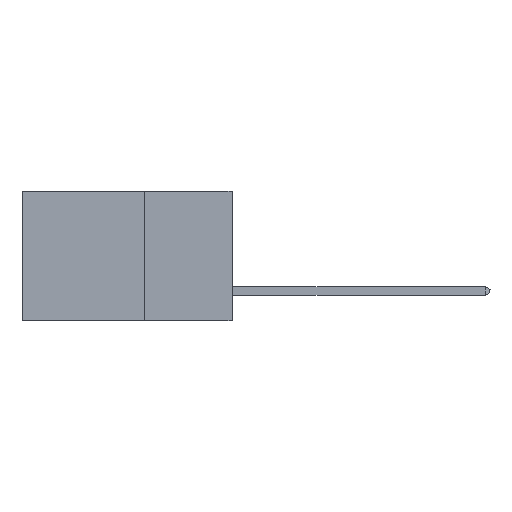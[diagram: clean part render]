
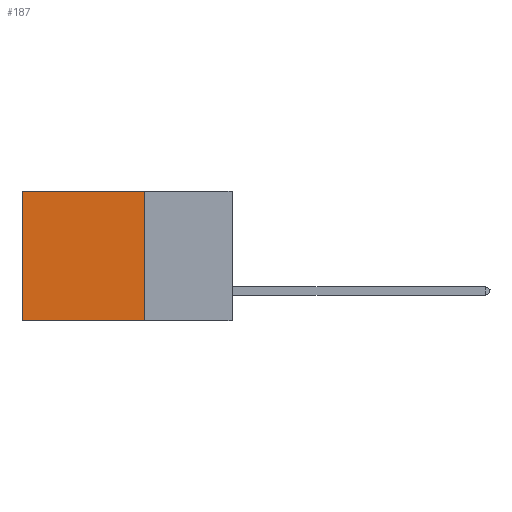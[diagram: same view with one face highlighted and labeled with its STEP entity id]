
A CAD part, left-side view. The second image highlights one B-rep face of the part: STEP entity #187.
In plain terms, the highlighted planar face has unit normal (-1, 0, 0).
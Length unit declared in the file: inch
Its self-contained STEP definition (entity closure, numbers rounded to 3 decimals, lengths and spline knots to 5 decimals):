
#187 = ADVANCED_FACE ( 'NONE', ( #5172 ), #18684, .F. ) ;
#511 = ORIENTED_EDGE ( 'NONE', *, *, #18909, .F. ) ;
#770 = VECTOR ( 'NONE', #10409, 39.37008 ) ;
#1009 = VECTOR ( 'NONE', #8245, 39.37008 ) ;
#1285 = CARTESIAN_POINT ( 'NONE',  ( 0.2875, 0.6, 0. ) ) ;
#1453 = CARTESIAN_POINT ( 'NONE',  ( 0.2875, 0.25, 0. ) ) ;
#2769 = VERTEX_POINT ( 'NONE', #27573 ) ;
#3596 = ORIENTED_EDGE ( 'NONE', *, *, #14658, .T. ) ;
#3694 = DIRECTION ( 'NONE',  ( 0., 1., 0. ) ) ;
#4223 = CARTESIAN_POINT ( 'NONE',  ( 0.2875, 0.6, -0.37 ) ) ;
#4776 = LINE ( 'NONE', #6081, #27392 ) ;
#5172 = FACE_OUTER_BOUND ( 'NONE', #27755, .T. ) ;
#5697 = CARTESIAN_POINT ( 'NONE',  ( 0.2875, 0.25, 0. ) ) ;
#5830 = VECTOR ( 'NONE', #24695, 39.37008 ) ;
#6081 = CARTESIAN_POINT ( 'NONE',  ( 0.2875, 0.25, -0.37 ) ) ;
#7143 = LINE ( 'NONE', #22536, #5830 ) ;
#7458 = VERTEX_POINT ( 'NONE', #11482 ) ;
#7791 = EDGE_CURVE ( 'NONE', #2769, #12988, #4776, .T. ) ;
#7856 = CARTESIAN_POINT ( 'NONE',  ( 0.2875, 0.25, 0. ) ) ;
#8245 = DIRECTION ( 'NONE',  ( 0., 0., -1. ) ) ;
#8642 = LINE ( 'NONE', #1453, #770 ) ;
#10409 = DIRECTION ( 'NONE',  ( 0., 0., -1. ) ) ;
#11482 = CARTESIAN_POINT ( 'NONE',  ( 0.2875, 0.6, 0. ) ) ;
#12988 = VERTEX_POINT ( 'NONE', #4223 ) ;
#14193 = LINE ( 'NONE', #1285, #1009 ) ;
#14499 = AXIS2_PLACEMENT_3D ( 'NONE', #5697, #20645, #20837 ) ;
#14658 = EDGE_CURVE ( 'NONE', #15773, #7458, #7143, .T. ) ;
#15773 = VERTEX_POINT ( 'NONE', #7856 ) ;
#17794 = ORIENTED_EDGE ( 'NONE', *, *, #21390, .T. ) ;
#18684 = PLANE ( 'NONE',  #14499 ) ;
#18825 = ORIENTED_EDGE ( 'NONE', *, *, #7791, .F. ) ;
#18909 = EDGE_CURVE ( 'NONE', #15773, #2769, #8642, .T. ) ;
#20645 = DIRECTION ( 'NONE',  ( 1., 0., 0. ) ) ;
#20837 = DIRECTION ( 'NONE',  ( 0., 0., -1. ) ) ;
#21390 = EDGE_CURVE ( 'NONE', #7458, #12988, #14193, .T. ) ;
#22536 = CARTESIAN_POINT ( 'NONE',  ( 0.2875, 0.25, 0. ) ) ;
#24695 = DIRECTION ( 'NONE',  ( 0., 1., 0. ) ) ;
#27392 = VECTOR ( 'NONE', #3694, 39.37008 ) ;
#27573 = CARTESIAN_POINT ( 'NONE',  ( 0.2875, 0.25, -0.37 ) ) ;
#27755 = EDGE_LOOP ( 'NONE', ( #17794, #18825, #511, #3596 ) ) ;
